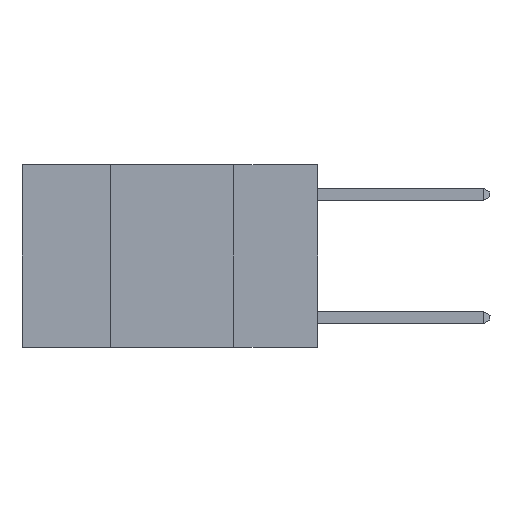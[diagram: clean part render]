
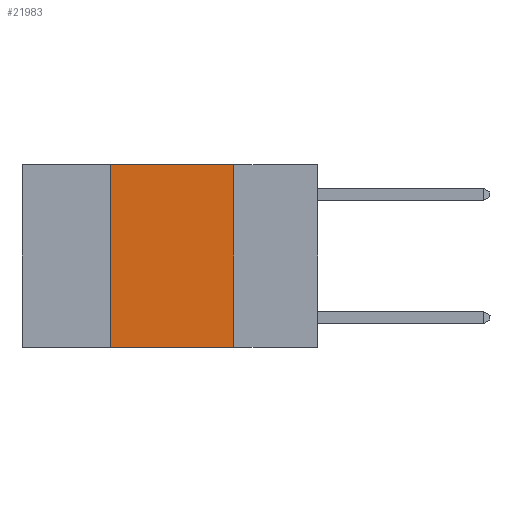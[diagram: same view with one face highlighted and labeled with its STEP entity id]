
A CAD part, left-side view. The second image highlights one B-rep face of the part: STEP entity #21983.
In plain terms, the highlighted planar face has unit normal (-1, 0, 0).
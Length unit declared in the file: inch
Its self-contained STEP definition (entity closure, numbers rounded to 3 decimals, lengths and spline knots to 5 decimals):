
#244 = DIRECTION ( 'NONE',  ( 0., 0., -1. ) ) ;
#523 = CARTESIAN_POINT ( 'NONE',  ( 0., 0.42, 0. ) ) ;
#569 = ORIENTED_EDGE ( 'NONE', *, *, #21720, .F. ) ;
#781 = ORIENTED_EDGE ( 'NONE', *, *, #14272, .F. ) ;
#858 = ORIENTED_EDGE ( 'NONE', *, *, #14904, .F. ) ;
#902 = ORIENTED_EDGE ( 'NONE', *, *, #21114, .T. ) ;
#1639 = LINE ( 'NONE', #1943, #17003 ) ;
#1811 = DIRECTION ( 'NONE',  ( 0., 0., 1. ) ) ;
#1943 = CARTESIAN_POINT ( 'NONE',  ( 0., 0.6, 0. ) ) ;
#2105 = LINE ( 'NONE', #16342, #22574 ) ;
#5887 = FACE_OUTER_BOUND ( 'NONE', #22371, .T. ) ;
#7207 = LINE ( 'NONE', #14515, #11955 ) ;
#7235 = DIRECTION ( 'NONE',  ( 1., 0., 0. ) ) ;
#7723 = VERTEX_POINT ( 'NONE', #18042 ) ;
#8307 = VERTEX_POINT ( 'NONE', #11611 ) ;
#11611 = CARTESIAN_POINT ( 'NONE',  ( 0., 0.42, -0.37 ) ) ;
#11955 = VECTOR ( 'NONE', #12495, 39.37008 ) ;
#12031 = DIRECTION ( 'NONE',  ( 0., -1., 0. ) ) ;
#12495 = DIRECTION ( 'NONE',  ( 0., -1., 0. ) ) ;
#13248 = PLANE ( 'NONE',  #22443 ) ;
#14272 = EDGE_CURVE ( 'NONE', #8307, #17437, #25055, .T. ) ;
#14515 = CARTESIAN_POINT ( 'NONE',  ( 0., 0.6, -0.37 ) ) ;
#14904 = EDGE_CURVE ( 'NONE', #17437, #7723, #1639, .T. ) ;
#15614 = CARTESIAN_POINT ( 'NONE',  ( 0., 0.17, -0.37 ) ) ;
#15796 = CARTESIAN_POINT ( 'NONE',  ( 0., 0.42, 0. ) ) ;
#16342 = CARTESIAN_POINT ( 'NONE',  ( 0., 0.17, 0. ) ) ;
#17003 = VECTOR ( 'NONE', #12031, 39.37008 ) ;
#17437 = VERTEX_POINT ( 'NONE', #523 ) ;
#18042 = CARTESIAN_POINT ( 'NONE',  ( 0., 0.17, 0. ) ) ;
#19153 = CARTESIAN_POINT ( 'NONE',  ( 0., 0.6, 0. ) ) ;
#19477 = VECTOR ( 'NONE', #1811, 39.37008 ) ;
#21087 = DIRECTION ( 'NONE',  ( 0., 0., -1. ) ) ;
#21114 = EDGE_CURVE ( 'NONE', #8307, #21468, #7207, .T. ) ;
#21468 = VERTEX_POINT ( 'NONE', #15614 ) ;
#21720 = EDGE_CURVE ( 'NONE', #7723, #21468, #2105, .T. ) ;
#21983 = ADVANCED_FACE ( 'NONE', ( #5887 ), #13248, .F. ) ;
#22371 = EDGE_LOOP ( 'NONE', ( #569, #858, #781, #902 ) ) ;
#22443 = AXIS2_PLACEMENT_3D ( 'NONE', #19153, #7235, #21087 ) ;
#22574 = VECTOR ( 'NONE', #244, 39.37008 ) ;
#25055 = LINE ( 'NONE', #15796, #19477 ) ;
